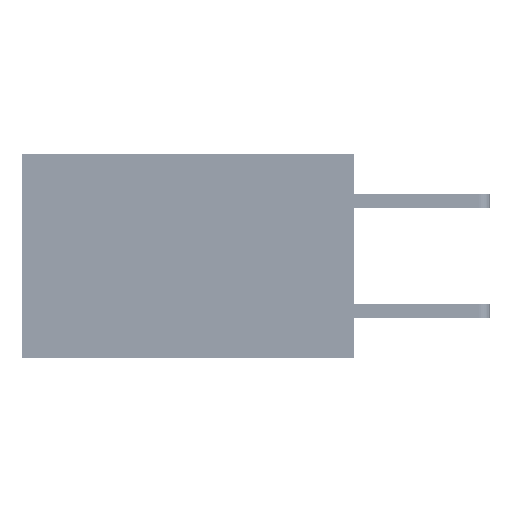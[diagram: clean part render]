
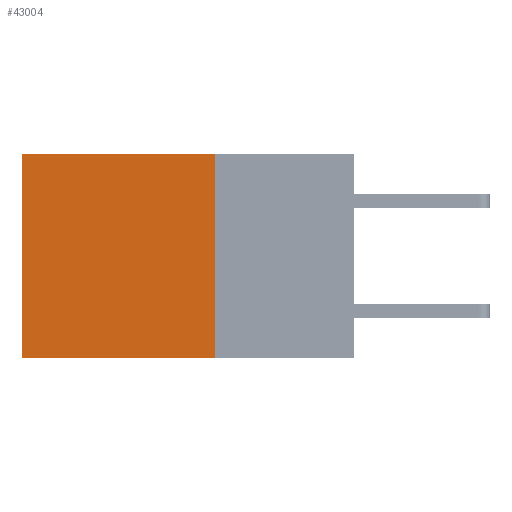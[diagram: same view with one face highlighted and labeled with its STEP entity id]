
A CAD part, left-side view. The second image highlights one B-rep face of the part: STEP entity #43004.
In plain terms, the highlighted planar face has unit normal (-1, 0, 0).
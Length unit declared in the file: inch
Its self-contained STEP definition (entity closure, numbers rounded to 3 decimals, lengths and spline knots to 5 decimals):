
#58 = VECTOR ( 'NONE', #34622, 39.37008 ) ;
#142 = EDGE_CURVE ( 'NONE', #3803, #21537, #42187, .T. ) ;
#268 = CARTESIAN_POINT ( 'NONE',  ( 0.2875, 0.25, -0.37 ) ) ;
#353 = AXIS2_PLACEMENT_3D ( 'NONE', #9012, #44851, #23501 ) ;
#3803 = VERTEX_POINT ( 'NONE', #10391 ) ;
#4244 = CARTESIAN_POINT ( 'NONE',  ( 0.2875, 0.6, 0. ) ) ;
#4859 = CARTESIAN_POINT ( 'NONE',  ( 0.2875, 0.25, 0. ) ) ;
#9012 = CARTESIAN_POINT ( 'NONE',  ( 0.2875, 0.25, 0. ) ) ;
#10391 = CARTESIAN_POINT ( 'NONE',  ( 0.2875, 0.25, 0. ) ) ;
#10805 = LINE ( 'NONE', #16541, #58 ) ;
#11467 = VECTOR ( 'NONE', #12844, 39.37008 ) ;
#12460 = VECTOR ( 'NONE', #17749, 39.37008 ) ;
#12844 = DIRECTION ( 'NONE',  ( 0., 1., 0. ) ) ;
#13206 = CARTESIAN_POINT ( 'NONE',  ( 0.2875, 0.6, -0.37 ) ) ;
#14130 = CARTESIAN_POINT ( 'NONE',  ( 0.2875, 0.25, 0. ) ) ;
#16541 = CARTESIAN_POINT ( 'NONE',  ( 0.2875, 0.6, 0. ) ) ;
#17749 = DIRECTION ( 'NONE',  ( 0., 1., 0. ) ) ;
#18471 = ORIENTED_EDGE ( 'NONE', *, *, #29871, .F. ) ;
#19959 = EDGE_LOOP ( 'NONE', ( #21968, #18471, #39976, #30648 ) ) ;
#21537 = VERTEX_POINT ( 'NONE', #4244 ) ;
#21968 = ORIENTED_EDGE ( 'NONE', *, *, #41703, .T. ) ;
#22958 = DIRECTION ( 'NONE',  ( 0., 0., -1. ) ) ;
#23501 = DIRECTION ( 'NONE',  ( 0., 0., -1. ) ) ;
#24296 = VECTOR ( 'NONE', #22958, 39.37008 ) ;
#25288 = FACE_OUTER_BOUND ( 'NONE', #19959, .T. ) ;
#29871 = EDGE_CURVE ( 'NONE', #42033, #46429, #40095, .T. ) ;
#30648 = ORIENTED_EDGE ( 'NONE', *, *, #142, .T. ) ;
#34403 = CARTESIAN_POINT ( 'NONE',  ( 0.2875, 0.25, -0.37 ) ) ;
#34622 = DIRECTION ( 'NONE',  ( 0., 0., -1. ) ) ;
#34980 = LINE ( 'NONE', #4859, #24296 ) ;
#37273 = EDGE_CURVE ( 'NONE', #3803, #42033, #34980, .T. ) ;
#39976 = ORIENTED_EDGE ( 'NONE', *, *, #37273, .F. ) ;
#40095 = LINE ( 'NONE', #34403, #11467 ) ;
#41333 = PLANE ( 'NONE',  #353 ) ;
#41703 = EDGE_CURVE ( 'NONE', #21537, #46429, #10805, .T. ) ;
#42033 = VERTEX_POINT ( 'NONE', #268 ) ;
#42187 = LINE ( 'NONE', #14130, #12460 ) ;
#43004 = ADVANCED_FACE ( 'NONE', ( #25288 ), #41333, .F. ) ;
#44851 = DIRECTION ( 'NONE',  ( 1., 0., 0. ) ) ;
#46429 = VERTEX_POINT ( 'NONE', #13206 ) ;
